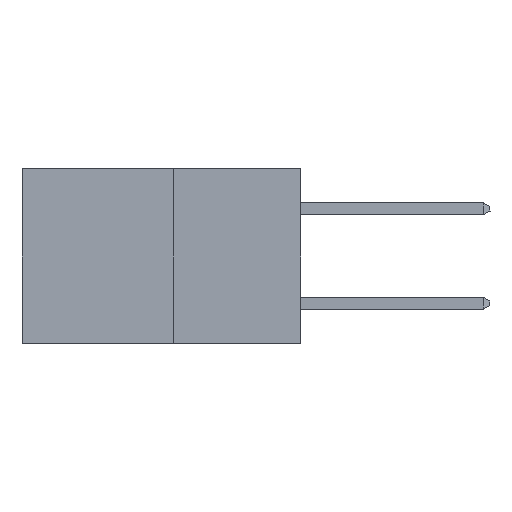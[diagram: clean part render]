
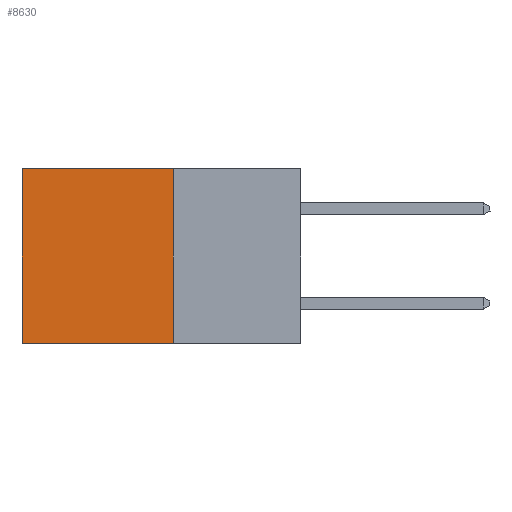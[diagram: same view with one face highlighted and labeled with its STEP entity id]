
A CAD part, left-side view. The second image highlights one B-rep face of the part: STEP entity #8630.
In plain terms, the highlighted planar face has unit normal (-1, 0, 0).
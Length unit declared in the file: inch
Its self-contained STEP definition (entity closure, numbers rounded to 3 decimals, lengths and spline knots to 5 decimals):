
#50 = LINE ( 'NONE', #22316, #6748 ) ;
#2178 = DIRECTION ( 'NONE',  ( 0., 1., 0. ) ) ;
#4464 = CARTESIAN_POINT ( 'NONE',  ( 0.277, 0.27, -0.37 ) ) ;
#5484 = EDGE_LOOP ( 'NONE', ( #6506, #19045, #11655, #35917 ) ) ;
#5678 = EDGE_CURVE ( 'NONE', #6619, #10023, #9636, .T. ) ;
#6506 = ORIENTED_EDGE ( 'NONE', *, *, #7782, .T. ) ;
#6619 = VERTEX_POINT ( 'NONE', #25738 ) ;
#6748 = VECTOR ( 'NONE', #30637, 39.37008 ) ;
#7042 = FACE_OUTER_BOUND ( 'NONE', #5484, .T. ) ;
#7287 = DIRECTION ( 'NONE',  ( 0., 0., -1. ) ) ;
#7782 = EDGE_CURVE ( 'NONE', #29882, #10023, #36152, .T. ) ;
#8630 = ADVANCED_FACE ( 'NONE', ( #7042 ), #32415, .F. ) ;
#9636 = LINE ( 'NONE', #16235, #16212 ) ;
#10023 = VERTEX_POINT ( 'NONE', #13454 ) ;
#10878 = VERTEX_POINT ( 'NONE', #14101 ) ;
#11655 = ORIENTED_EDGE ( 'NONE', *, *, #34549, .F. ) ;
#12269 = DIRECTION ( 'NONE',  ( 0., 0., -1. ) ) ;
#12769 = DIRECTION ( 'NONE',  ( 0., 1., 0. ) ) ;
#12995 = LINE ( 'NONE', #35155, #18703 ) ;
#13454 = CARTESIAN_POINT ( 'NONE',  ( 0.277, 0.59, -0.37 ) ) ;
#14060 = AXIS2_PLACEMENT_3D ( 'NONE', #4464, #24098, #7287 ) ;
#14101 = CARTESIAN_POINT ( 'NONE',  ( 0.277, 0.27, 0. ) ) ;
#16212 = VECTOR ( 'NONE', #2178, 39.37008 ) ;
#16235 = CARTESIAN_POINT ( 'NONE',  ( 0.277, 0.27, -0.37 ) ) ;
#18703 = VECTOR ( 'NONE', #12769, 39.37008 ) ;
#19045 = ORIENTED_EDGE ( 'NONE', *, *, #5678, .F. ) ;
#20448 = VECTOR ( 'NONE', #12269, 39.37008 ) ;
#22316 = CARTESIAN_POINT ( 'NONE',  ( 0.277, 0.27, -0.37 ) ) ;
#23471 = EDGE_CURVE ( 'NONE', #10878, #29882, #12995, .T. ) ;
#24098 = DIRECTION ( 'NONE',  ( 1., 0., 0. ) ) ;
#25738 = CARTESIAN_POINT ( 'NONE',  ( 0.277, 0.27, -0.37 ) ) ;
#26377 = CARTESIAN_POINT ( 'NONE',  ( 0.277, 0.59, -0.37 ) ) ;
#29882 = VERTEX_POINT ( 'NONE', #30564 ) ;
#30564 = CARTESIAN_POINT ( 'NONE',  ( 0.277, 0.59, 0. ) ) ;
#30637 = DIRECTION ( 'NONE',  ( 0., 0., -1. ) ) ;
#32415 = PLANE ( 'NONE',  #14060 ) ;
#34549 = EDGE_CURVE ( 'NONE', #10878, #6619, #50, .T. ) ;
#35155 = CARTESIAN_POINT ( 'NONE',  ( 0.277, 0.27, 0. ) ) ;
#35917 = ORIENTED_EDGE ( 'NONE', *, *, #23471, .T. ) ;
#36152 = LINE ( 'NONE', #26377, #20448 ) ;
